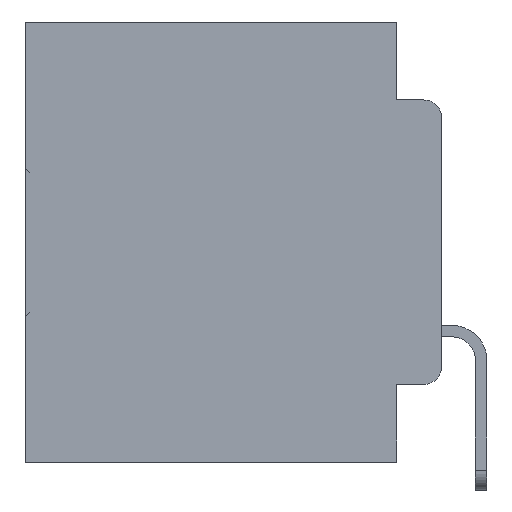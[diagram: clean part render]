
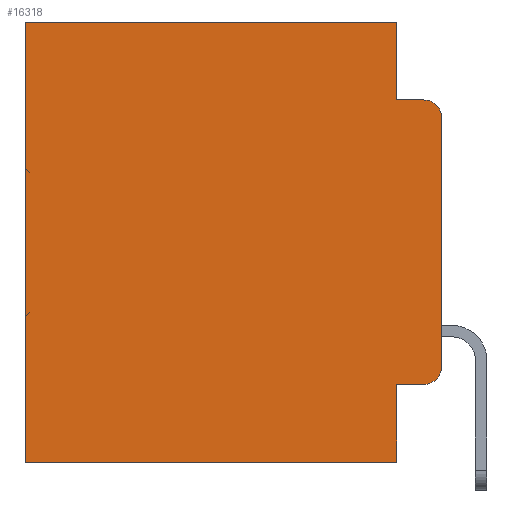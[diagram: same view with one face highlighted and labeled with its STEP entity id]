
A CAD part, left-side view. The second image highlights one B-rep face of the part: STEP entity #16318.
In plain terms, the highlighted planar face has unit normal (-1, 0, 0).
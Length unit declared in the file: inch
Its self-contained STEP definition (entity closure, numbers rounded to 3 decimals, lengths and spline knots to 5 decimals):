
#95 = LINE ( 'NONE', #7813, #13566 ) ;
#431 = EDGE_CURVE ( 'NONE', #8437, #2700, #16158, .T. ) ;
#1235 = PLANE ( 'NONE',  #8160 ) ;
#1552 = LINE ( 'NONE', #28983, #28404 ) ;
#2077 = VERTEX_POINT ( 'NONE', #32466 ) ;
#2134 = AXIS2_PLACEMENT_3D ( 'NONE', #24565, #9065, #27062 ) ;
#2272 = EDGE_CURVE ( 'NONE', #2700, #2077, #27892, .T. ) ;
#2700 = VERTEX_POINT ( 'NONE', #19699 ) ;
#3629 = VERTEX_POINT ( 'NONE', #26230 ) ;
#4740 = VERTEX_POINT ( 'NONE', #10182 ) ;
#5457 = LINE ( 'NONE', #30145, #32032 ) ;
#6176 = ORIENTED_EDGE ( 'NONE', *, *, #17228, .T. ) ;
#6737 = CARTESIAN_POINT ( 'NONE',  ( 0.298, 0., 0. ) ) ;
#7381 = VECTOR ( 'NONE', #13821, 39.37008 ) ;
#7430 = CARTESIAN_POINT ( 'NONE',  ( 0.298, 0.051, 0. ) ) ;
#7813 = CARTESIAN_POINT ( 'NONE',  ( 0.298, 0.051, -0.4115 ) ) ;
#8160 = AXIS2_PLACEMENT_3D ( 'NONE', #6737, #24863, #9355 ) ;
#8301 = VECTOR ( 'NONE', #21395, 39.37008 ) ;
#8337 = DIRECTION ( 'NONE',  ( 0., 0., -1. ) ) ;
#8437 = VERTEX_POINT ( 'NONE', #7430 ) ;
#8746 = LINE ( 'NONE', #23863, #22601 ) ;
#8778 = CARTESIAN_POINT ( 'NONE',  ( 0.298, 0.051, -0.0885 ) ) ;
#9065 = DIRECTION ( 'NONE',  ( -1., 0., 0. ) ) ;
#9132 = VECTOR ( 'NONE', #25469, 39.37008 ) ;
#9355 = DIRECTION ( 'NONE',  ( 0., 0., -1. ) ) ;
#9466 = VERTEX_POINT ( 'NONE', #29353 ) ;
#9539 = VERTEX_POINT ( 'NONE', #22149 ) ;
#10182 = CARTESIAN_POINT ( 'NONE',  ( 0.298, 0.473, -0.5 ) ) ;
#10465 = DIRECTION ( 'NONE',  ( 0., -1., 0. ) ) ;
#11279 = EDGE_CURVE ( 'NONE', #3629, #2077, #16162, .T. ) ;
#11525 = CARTESIAN_POINT ( 'NONE',  ( 0.298, 0.051, -0.4115 ) ) ;
#12325 = CIRCLE ( 'NONE', #20236, 0.02 ) ;
#12344 = CARTESIAN_POINT ( 'NONE',  ( 0.298, 0.473, 0. ) ) ;
#12359 = ORIENTED_EDGE ( 'NONE', *, *, #14840, .F. ) ;
#13302 = EDGE_CURVE ( 'NONE', #9539, #4740, #5457, .T. ) ;
#13566 = VECTOR ( 'NONE', #10465, 39.37008 ) ;
#13821 = DIRECTION ( 'NONE',  ( 0., -1., 0. ) ) ;
#14013 = ORIENTED_EDGE ( 'NONE', *, *, #30736, .T. ) ;
#14410 = CARTESIAN_POINT ( 'NONE',  ( 0.298, 0.473, 0. ) ) ;
#14840 = EDGE_CURVE ( 'NONE', #3629, #9466, #22145, .T. ) ;
#14993 = DIRECTION ( 'NONE',  ( 0., 1., 0. ) ) ;
#15755 = DIRECTION ( 'NONE',  ( -1., 0., 0. ) ) ;
#16158 = LINE ( 'NONE', #30880, #9132 ) ;
#16162 = CIRCLE ( 'NONE', #2134, 0.02 ) ;
#16318 = ADVANCED_FACE ( 'NONE', ( #23235 ), #1235, .F. ) ;
#16485 = ORIENTED_EDGE ( 'NONE', *, *, #13302, .F. ) ;
#17228 = EDGE_CURVE ( 'NONE', #26995, #9466, #12325, .T. ) ;
#18571 = VERTEX_POINT ( 'NONE', #11525 ) ;
#18885 = CARTESIAN_POINT ( 'NONE',  ( 0.298, 0., 0. ) ) ;
#18966 = EDGE_CURVE ( 'NONE', #18571, #26995, #95, .T. ) ;
#19305 = ORIENTED_EDGE ( 'NONE', *, *, #11279, .T. ) ;
#19338 = ORIENTED_EDGE ( 'NONE', *, *, #18966, .T. ) ;
#19699 = CARTESIAN_POINT ( 'NONE',  ( 0.298, 0.051, -0.0885 ) ) ;
#20096 = VERTEX_POINT ( 'NONE', #12344 ) ;
#20236 = AXIS2_PLACEMENT_3D ( 'NONE', #30894, #15755, #33413 ) ;
#20873 = ORIENTED_EDGE ( 'NONE', *, *, #23459, .T. ) ;
#21325 = EDGE_LOOP ( 'NONE', ( #12359, #19305, #32279, #26772, #20873, #14013, #16485, #33461, #19338, #6176 ) ) ;
#21395 = DIRECTION ( 'NONE',  ( 0., 0., -1. ) ) ;
#21561 = CARTESIAN_POINT ( 'NONE',  ( 0.298, 0.02, -0.4115 ) ) ;
#22145 = LINE ( 'NONE', #18885, #8301 ) ;
#22149 = CARTESIAN_POINT ( 'NONE',  ( 0.298, 0.051, -0.5 ) ) ;
#22170 = DIRECTION ( 'NONE',  ( 0., 0., -1. ) ) ;
#22341 = EDGE_CURVE ( 'NONE', #18571, #9539, #8746, .T. ) ;
#22601 = VECTOR ( 'NONE', #8337, 39.37008 ) ;
#23235 = FACE_OUTER_BOUND ( 'NONE', #21325, .T. ) ;
#23459 = EDGE_CURVE ( 'NONE', #8437, #20096, #1552, .T. ) ;
#23863 = CARTESIAN_POINT ( 'NONE',  ( 0.298, 0.051, 0. ) ) ;
#24565 = CARTESIAN_POINT ( 'NONE',  ( 0.298, 0.02, -0.1085 ) ) ;
#24863 = DIRECTION ( 'NONE',  ( 1., 0., 0. ) ) ;
#25469 = DIRECTION ( 'NONE',  ( 0., 0., -1. ) ) ;
#26230 = CARTESIAN_POINT ( 'NONE',  ( 0.298, 0., -0.1085 ) ) ;
#26593 = DIRECTION ( 'NONE',  ( 0., 1., 0. ) ) ;
#26772 = ORIENTED_EDGE ( 'NONE', *, *, #431, .F. ) ;
#26995 = VERTEX_POINT ( 'NONE', #21561 ) ;
#27062 = DIRECTION ( 'NONE',  ( 0., 0., -1. ) ) ;
#27892 = LINE ( 'NONE', #8778, #7381 ) ;
#28404 = VECTOR ( 'NONE', #26593, 39.37008 ) ;
#28983 = CARTESIAN_POINT ( 'NONE',  ( 0.298, 0., 0. ) ) ;
#29353 = CARTESIAN_POINT ( 'NONE',  ( 0.298, 0., -0.3915 ) ) ;
#29490 = VECTOR ( 'NONE', #22170, 39.37008 ) ;
#30145 = CARTESIAN_POINT ( 'NONE',  ( 0.298, 0., -0.5 ) ) ;
#30303 = LINE ( 'NONE', #14410, #29490 ) ;
#30736 = EDGE_CURVE ( 'NONE', #20096, #4740, #30303, .T. ) ;
#30880 = CARTESIAN_POINT ( 'NONE',  ( 0.298, 0.051, 0. ) ) ;
#30894 = CARTESIAN_POINT ( 'NONE',  ( 0.298, 0.02, -0.3915 ) ) ;
#32032 = VECTOR ( 'NONE', #14993, 39.37008 ) ;
#32279 = ORIENTED_EDGE ( 'NONE', *, *, #2272, .F. ) ;
#32466 = CARTESIAN_POINT ( 'NONE',  ( 0.298, 0.02, -0.0885 ) ) ;
#33413 = DIRECTION ( 'NONE',  ( 0., 0., -1. ) ) ;
#33461 = ORIENTED_EDGE ( 'NONE', *, *, #22341, .F. ) ;
